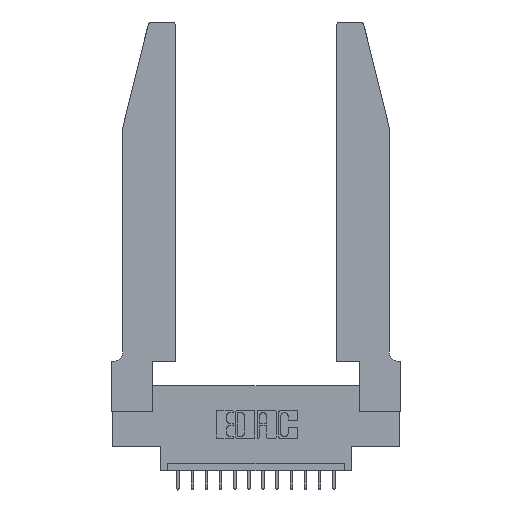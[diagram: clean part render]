
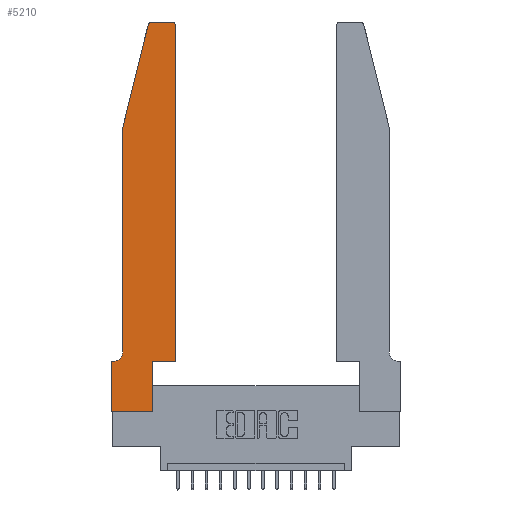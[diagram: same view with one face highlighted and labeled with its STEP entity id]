
A CAD part, top view. The second image highlights one B-rep face of the part: STEP entity #5210.
In plain terms, the highlighted planar face has unit normal (0, 0, 1).
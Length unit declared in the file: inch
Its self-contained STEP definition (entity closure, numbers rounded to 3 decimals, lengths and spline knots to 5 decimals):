
#274 = AXIS2_PLACEMENT_3D ( 'NONE', #14390, #1891, #7636 ) ;
#665 = VECTOR ( 'NONE', #14990, 39.37008 ) ;
#670 = VECTOR ( 'NONE', #7225, 39.37008 ) ;
#729 = DIRECTION ( 'NONE',  ( 0., 1., 0. ) ) ;
#969 = CARTESIAN_POINT ( 'NONE',  ( 0.0055, 0.35, 0.37 ) ) ;
#1049 = LINE ( 'NONE', #6600, #14226 ) ;
#1460 = DIRECTION ( 'NONE',  ( 0., 1., 0. ) ) ;
#1520 = AXIS2_PLACEMENT_3D ( 'NONE', #8960, #3309, #13145 ) ;
#1545 = CIRCLE ( 'NONE', #10550, 0.03 ) ;
#1777 = LINE ( 'NONE', #15387, #7738 ) ;
#1796 = CIRCLE ( 'NONE', #1520, 0.03 ) ;
#1891 = DIRECTION ( 'NONE',  ( 0., 0., 1. ) ) ;
#2051 = VERTEX_POINT ( 'NONE', #969 ) ;
#2224 = CARTESIAN_POINT ( 'NONE',  ( 0.4505, 2.72, 0.37 ) ) ;
#2320 = DIRECTION ( 'NONE',  ( -1., 0., 0. ) ) ;
#2627 = EDGE_CURVE ( 'NONE', #3039, #16901, #4104, .T. ) ;
#2918 = CARTESIAN_POINT ( 'NONE',  ( 0.4505, 0.35, 0.37 ) ) ;
#3039 = VERTEX_POINT ( 'NONE', #14955 ) ;
#3166 = CARTESIAN_POINT ( 'NONE',  ( 0.25487, 2.72718, 0.37 ) ) ;
#3309 = DIRECTION ( 'NONE',  ( 0., 0., 1. ) ) ;
#3411 = VERTEX_POINT ( 'NONE', #16834 ) ;
#3878 = DIRECTION ( 'NONE',  ( 0., -1., 0. ) ) ;
#4104 = LINE ( 'NONE', #2918, #7224 ) ;
#4257 = DIRECTION ( 'NONE',  ( 1., 0., 0. ) ) ;
#4367 = EDGE_CURVE ( 'NONE', #5758, #10793, #1049, .T. ) ;
#5110 = LINE ( 'NONE', #10682, #665 ) ;
#5210 = ADVANCED_FACE ( 'NONE', ( #10189 ), #13208, .T. ) ;
#5264 = ORIENTED_EDGE ( 'NONE', *, *, #17993, .T. ) ;
#5306 = VECTOR ( 'NONE', #6068, 39.37008 ) ;
#5314 = VERTEX_POINT ( 'NONE', #14578 ) ;
#5431 = ORIENTED_EDGE ( 'NONE', *, *, #4367, .T. ) ;
#5485 = CARTESIAN_POINT ( 'NONE',  ( 0., 0.35, 0.37 ) ) ;
#5532 = DIRECTION ( 'NONE',  ( 0., 0., -1. ) ) ;
#5758 = VERTEX_POINT ( 'NONE', #5485 ) ;
#5828 = CARTESIAN_POINT ( 'NONE',  ( 0.4205, 2.72, 0.37 ) ) ;
#6068 = DIRECTION ( 'NONE',  ( 1., 0., 0. ) ) ;
#6156 = VERTEX_POINT ( 'NONE', #15246 ) ;
#6175 = CIRCLE ( 'NONE', #16395, 0.07 ) ;
#6220 = CARTESIAN_POINT ( 'NONE',  ( 0.0755, 0.35, 0.37 ) ) ;
#6600 = CARTESIAN_POINT ( 'NONE',  ( 0., 0., 0.37 ) ) ;
#6709 = ORIENTED_EDGE ( 'NONE', *, *, #10199, .T. ) ;
#7135 = CARTESIAN_POINT ( 'NONE',  ( 0.2605, 2.75, 0.37 ) ) ;
#7224 = VECTOR ( 'NONE', #1460, 39.37008 ) ;
#7225 = DIRECTION ( 'NONE',  ( -1., 0., 0. ) ) ;
#7311 = LINE ( 'NONE', #7135, #670 ) ;
#7373 = VERTEX_POINT ( 'NONE', #9329 ) ;
#7411 = ORIENTED_EDGE ( 'NONE', *, *, #13630, .T. ) ;
#7636 = DIRECTION ( 'NONE',  ( 1., 0., 0. ) ) ;
#7738 = VECTOR ( 'NONE', #16935, 39.37008 ) ;
#7762 = ORIENTED_EDGE ( 'NONE', *, *, #7930, .T. ) ;
#7916 = ORIENTED_EDGE ( 'NONE', *, *, #17337, .T. ) ;
#7930 = EDGE_CURVE ( 'NONE', #3411, #13513, #9202, .T. ) ;
#8186 = LINE ( 'NONE', #8284, #14676 ) ;
#8191 = VERTEX_POINT ( 'NONE', #3166 ) ;
#8284 = CARTESIAN_POINT ( 'NONE',  ( 0., 0., 0.37 ) ) ;
#8303 = EDGE_CURVE ( 'NONE', #13513, #3039, #8909, .T. ) ;
#8595 = ORIENTED_EDGE ( 'NONE', *, *, #8303, .T. ) ;
#8684 = EDGE_LOOP ( 'NONE', ( #13148, #6709, #7411, #13789, #12964, #5264, #5431, #7916, #7762, #8595, #15091, #16164 ) ) ;
#8909 = LINE ( 'NONE', #9003, #5306 ) ;
#8960 = CARTESIAN_POINT ( 'NONE',  ( 0.284, 2.72, 0.37 ) ) ;
#9003 = CARTESIAN_POINT ( 'NONE',  ( 0.4505, 0.35, 0.37 ) ) ;
#9202 = LINE ( 'NONE', #14776, #16081 ) ;
#9329 = CARTESIAN_POINT ( 'NONE',  ( 0.284, 2.75, 0.37 ) ) ;
#9443 = DIRECTION ( 'NONE',  ( 0., 0., 1. ) ) ;
#9466 = CARTESIAN_POINT ( 'NONE',  ( 0.2865, 0.35, 0.37 ) ) ;
#10189 = FACE_OUTER_BOUND ( 'NONE', #8684, .T. ) ;
#10199 = EDGE_CURVE ( 'NONE', #7373, #8191, #1796, .T. ) ;
#10390 = EDGE_CURVE ( 'NONE', #5314, #6156, #5110, .T. ) ;
#10550 = AXIS2_PLACEMENT_3D ( 'NONE', #5828, #9443, #15015 ) ;
#10682 = CARTESIAN_POINT ( 'NONE',  ( 0.0755, 2., 0.37 ) ) ;
#10793 = VERTEX_POINT ( 'NONE', #17955 ) ;
#12455 = CARTESIAN_POINT ( 'NONE',  ( 0.0055, 0.42, 0.37 ) ) ;
#12964 = ORIENTED_EDGE ( 'NONE', *, *, #16330, .T. ) ;
#13145 = DIRECTION ( 'NONE',  ( 1., 0., 0. ) ) ;
#13148 = ORIENTED_EDGE ( 'NONE', *, *, #16865, .T. ) ;
#13208 = PLANE ( 'NONE',  #274 ) ;
#13347 = LINE ( 'NONE', #6220, #14387 ) ;
#13513 = VERTEX_POINT ( 'NONE', #9466 ) ;
#13630 = EDGE_CURVE ( 'NONE', #8191, #5314, #1777, .T. ) ;
#13661 = DIRECTION ( 'NONE',  ( -1., 0., 0. ) ) ;
#13789 = ORIENTED_EDGE ( 'NONE', *, *, #10390, .T. ) ;
#14226 = VECTOR ( 'NONE', #3878, 39.37008 ) ;
#14371 = CARTESIAN_POINT ( 'NONE',  ( 0.4205, 2.75, 0.37 ) ) ;
#14387 = VECTOR ( 'NONE', #2320, 39.37008 ) ;
#14390 = CARTESIAN_POINT ( 'NONE',  ( 0., 0.35, 0.37 ) ) ;
#14578 = CARTESIAN_POINT ( 'NONE',  ( 0.0755, 2., 0.37 ) ) ;
#14676 = VECTOR ( 'NONE', #4257, 39.37008 ) ;
#14776 = CARTESIAN_POINT ( 'NONE',  ( 0.2865, 0.35, 0.37 ) ) ;
#14955 = CARTESIAN_POINT ( 'NONE',  ( 0.4505, 0.35, 0.37 ) ) ;
#14990 = DIRECTION ( 'NONE',  ( 0., -1., 0. ) ) ;
#15015 = DIRECTION ( 'NONE',  ( 1., 0., 0. ) ) ;
#15091 = ORIENTED_EDGE ( 'NONE', *, *, #2627, .T. ) ;
#15246 = CARTESIAN_POINT ( 'NONE',  ( 0.0755, 0.42, 0.37 ) ) ;
#15387 = CARTESIAN_POINT ( 'NONE',  ( 0.0755, 2., 0.37 ) ) ;
#15427 = EDGE_CURVE ( 'NONE', #16901, #16447, #1545, .T. ) ;
#16081 = VECTOR ( 'NONE', #729, 39.37008 ) ;
#16164 = ORIENTED_EDGE ( 'NONE', *, *, #15427, .T. ) ;
#16330 = EDGE_CURVE ( 'NONE', #6156, #2051, #6175, .T. ) ;
#16395 = AXIS2_PLACEMENT_3D ( 'NONE', #12455, #5532, #13661 ) ;
#16447 = VERTEX_POINT ( 'NONE', #14371 ) ;
#16834 = CARTESIAN_POINT ( 'NONE',  ( 0.2865, 0., 0.37 ) ) ;
#16865 = EDGE_CURVE ( 'NONE', #16447, #7373, #7311, .T. ) ;
#16901 = VERTEX_POINT ( 'NONE', #2224 ) ;
#16935 = DIRECTION ( 'NONE',  ( -0.239, -0.971, 0. ) ) ;
#17337 = EDGE_CURVE ( 'NONE', #10793, #3411, #8186, .T. ) ;
#17955 = CARTESIAN_POINT ( 'NONE',  ( 0., 0., 0.37 ) ) ;
#17993 = EDGE_CURVE ( 'NONE', #2051, #5758, #13347, .T. ) ;
